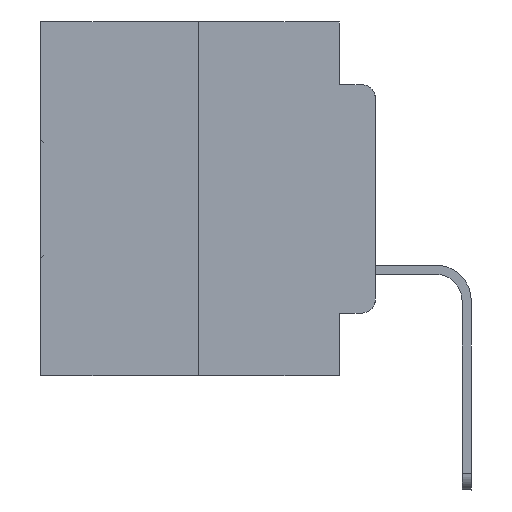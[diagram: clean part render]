
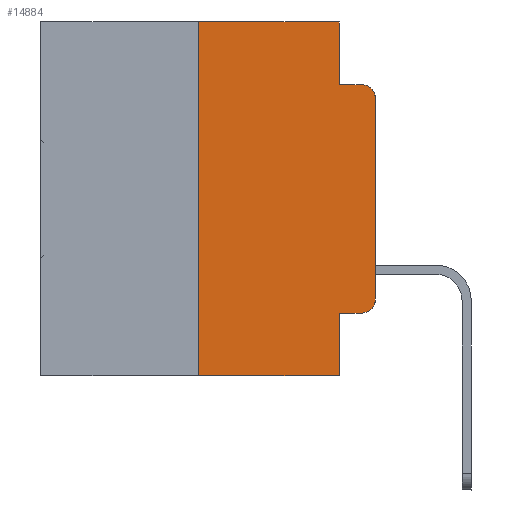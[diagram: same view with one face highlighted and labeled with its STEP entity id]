
A CAD part, left-side view. The second image highlights one B-rep face of the part: STEP entity #14884.
In plain terms, the highlighted planar face has unit normal (-1, 0, 0).
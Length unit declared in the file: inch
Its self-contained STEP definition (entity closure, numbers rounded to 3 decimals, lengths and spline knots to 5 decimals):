
#622 = CARTESIAN_POINT ( 'NONE',  ( 0., 0.02, -0.4115 ) ) ;
#786 = VERTEX_POINT ( 'NONE', #31314 ) ;
#855 = AXIS2_PLACEMENT_3D ( 'NONE', #19048, #6980, #11968 ) ;
#1511 = ORIENTED_EDGE ( 'NONE', *, *, #4835, .T. ) ;
#1875 = VECTOR ( 'NONE', #16800, 39.37008 ) ;
#1969 = VECTOR ( 'NONE', #29605, 39.37008 ) ;
#2345 = CARTESIAN_POINT ( 'NONE',  ( 0., 0., 0. ) ) ;
#2546 = EDGE_LOOP ( 'NONE', ( #24808, #30862, #21999, #8982, #15795, #23987, #19765, #6021, #1511, #23476 ) ) ;
#2719 = CARTESIAN_POINT ( 'NONE',  ( 0., 0.473, -0.5 ) ) ;
#2843 = CARTESIAN_POINT ( 'NONE',  ( 0., 0.051, 0. ) ) ;
#2876 = CARTESIAN_POINT ( 'NONE',  ( 0., 0., -0.3915 ) ) ;
#3572 = LINE ( 'NONE', #4710, #25563 ) ;
#3862 = VECTOR ( 'NONE', #17915, 39.37008 ) ;
#4505 = VERTEX_POINT ( 'NONE', #17971 ) ;
#4668 = CARTESIAN_POINT ( 'NONE',  ( 0., 0.051, -0.0885 ) ) ;
#4710 = CARTESIAN_POINT ( 'NONE',  ( 0., 0.051, 0. ) ) ;
#4835 = EDGE_CURVE ( 'NONE', #23397, #5030, #5999, .T. ) ;
#5030 = VERTEX_POINT ( 'NONE', #622 ) ;
#5070 = CARTESIAN_POINT ( 'NONE',  ( 0., 0.051, -0.0885 ) ) ;
#5228 = DIRECTION ( 'NONE',  ( 0., 0., -1. ) ) ;
#5999 = LINE ( 'NONE', #21764, #1875 ) ;
#6021 = ORIENTED_EDGE ( 'NONE', *, *, #11943, .F. ) ;
#6064 = EDGE_CURVE ( 'NONE', #786, #8302, #14110, .T. ) ;
#6980 = DIRECTION ( 'NONE',  ( -1., 0., 0. ) ) ;
#7361 = CARTESIAN_POINT ( 'NONE',  ( 0., 0.051, -0.4115 ) ) ;
#8302 = VERTEX_POINT ( 'NONE', #29918 ) ;
#8386 = LINE ( 'NONE', #27177, #1969 ) ;
#8982 = ORIENTED_EDGE ( 'NONE', *, *, #30840, .F. ) ;
#9141 = LINE ( 'NONE', #27568, #3862 ) ;
#9937 = DIRECTION ( 'NONE',  ( 0., -1., 0. ) ) ;
#10207 = PLANE ( 'NONE',  #14252 ) ;
#10420 = VECTOR ( 'NONE', #12191, 39.37008 ) ;
#10850 = EDGE_CURVE ( 'NONE', #13520, #786, #24864, .T. ) ;
#10861 = CARTESIAN_POINT ( 'NONE',  ( 0., 0.25, 0. ) ) ;
#10947 = VERTEX_POINT ( 'NONE', #4668 ) ;
#11492 = LINE ( 'NONE', #2719, #25179 ) ;
#11736 = VERTEX_POINT ( 'NONE', #2843 ) ;
#11943 = EDGE_CURVE ( 'NONE', #23397, #29598, #3572, .T. ) ;
#11968 = DIRECTION ( 'NONE',  ( 0., 0., -1. ) ) ;
#12191 = DIRECTION ( 'NONE',  ( 0., 0., 1. ) ) ;
#12386 = EDGE_CURVE ( 'NONE', #22904, #29598, #11492, .T. ) ;
#13520 = VERTEX_POINT ( 'NONE', #2876 ) ;
#13896 = LINE ( 'NONE', #5070, #27538 ) ;
#13921 = CARTESIAN_POINT ( 'NONE',  ( 0., 0.02, -0.3915 ) ) ;
#14110 = CIRCLE ( 'NONE', #855, 0.02 ) ;
#14252 = AXIS2_PLACEMENT_3D ( 'NONE', #21947, #29282, #5228 ) ;
#14393 = CARTESIAN_POINT ( 'NONE',  ( 0., 0.25, -0.5 ) ) ;
#14884 = ADVANCED_FACE ( 'NONE', ( #16291 ), #10207, .F. ) ;
#15507 = DIRECTION ( 'NONE',  ( 0., 0., 1. ) ) ;
#15795 = ORIENTED_EDGE ( 'NONE', *, *, #30802, .F. ) ;
#16291 = FACE_OUTER_BOUND ( 'NONE', #2546, .T. ) ;
#16800 = DIRECTION ( 'NONE',  ( 0., -1., 0. ) ) ;
#17915 = DIRECTION ( 'NONE',  ( 0., 0., -1. ) ) ;
#17971 = CARTESIAN_POINT ( 'NONE',  ( 0., 0.25, 0. ) ) ;
#18333 = EDGE_CURVE ( 'NONE', #5030, #13520, #27652, .T. ) ;
#19048 = CARTESIAN_POINT ( 'NONE',  ( 0., 0.02, -0.1085 ) ) ;
#19765 = ORIENTED_EDGE ( 'NONE', *, *, #12386, .T. ) ;
#21764 = CARTESIAN_POINT ( 'NONE',  ( 0., 0.051, -0.4115 ) ) ;
#21947 = CARTESIAN_POINT ( 'NONE',  ( 0., 0.473, 0. ) ) ;
#21999 = ORIENTED_EDGE ( 'NONE', *, *, #28039, .F. ) ;
#22682 = VECTOR ( 'NONE', #15507, 39.37008 ) ;
#22904 = VERTEX_POINT ( 'NONE', #14393 ) ;
#23397 = VERTEX_POINT ( 'NONE', #7361 ) ;
#23458 = LINE ( 'NONE', #10861, #22682 ) ;
#23476 = ORIENTED_EDGE ( 'NONE', *, *, #18333, .T. ) ;
#23559 = EDGE_CURVE ( 'NONE', #22904, #4505, #23458, .T. ) ;
#23767 = DIRECTION ( 'NONE',  ( 0., 0., -1. ) ) ;
#23987 = ORIENTED_EDGE ( 'NONE', *, *, #23559, .F. ) ;
#24708 = CARTESIAN_POINT ( 'NONE',  ( 0., 0.051, -0.5 ) ) ;
#24808 = ORIENTED_EDGE ( 'NONE', *, *, #10850, .T. ) ;
#24864 = LINE ( 'NONE', #2345, #10420 ) ;
#25179 = VECTOR ( 'NONE', #26977, 39.37008 ) ;
#25563 = VECTOR ( 'NONE', #26440, 39.37008 ) ;
#25922 = DIRECTION ( 'NONE',  ( -1., 0., 0. ) ) ;
#26440 = DIRECTION ( 'NONE',  ( 0., 0., -1. ) ) ;
#26977 = DIRECTION ( 'NONE',  ( 0., -1., 0. ) ) ;
#27177 = CARTESIAN_POINT ( 'NONE',  ( 0., 0.473, 0. ) ) ;
#27538 = VECTOR ( 'NONE', #9937, 39.37008 ) ;
#27568 = CARTESIAN_POINT ( 'NONE',  ( 0., 0.051, 0. ) ) ;
#27652 = CIRCLE ( 'NONE', #29583, 0.02 ) ;
#28039 = EDGE_CURVE ( 'NONE', #10947, #8302, #13896, .T. ) ;
#29282 = DIRECTION ( 'NONE',  ( 1., 0., 0. ) ) ;
#29583 = AXIS2_PLACEMENT_3D ( 'NONE', #13921, #25922, #23767 ) ;
#29598 = VERTEX_POINT ( 'NONE', #24708 ) ;
#29605 = DIRECTION ( 'NONE',  ( 0., -1., 0. ) ) ;
#29918 = CARTESIAN_POINT ( 'NONE',  ( 0., 0.02, -0.0885 ) ) ;
#30802 = EDGE_CURVE ( 'NONE', #4505, #11736, #8386, .T. ) ;
#30840 = EDGE_CURVE ( 'NONE', #11736, #10947, #9141, .T. ) ;
#30862 = ORIENTED_EDGE ( 'NONE', *, *, #6064, .T. ) ;
#31314 = CARTESIAN_POINT ( 'NONE',  ( 0., 0., -0.1085 ) ) ;
